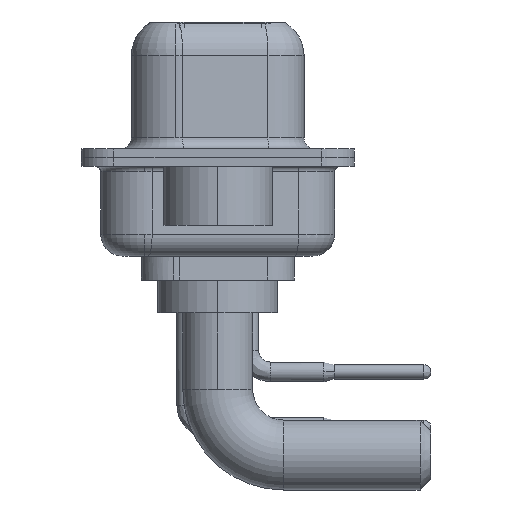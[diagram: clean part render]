
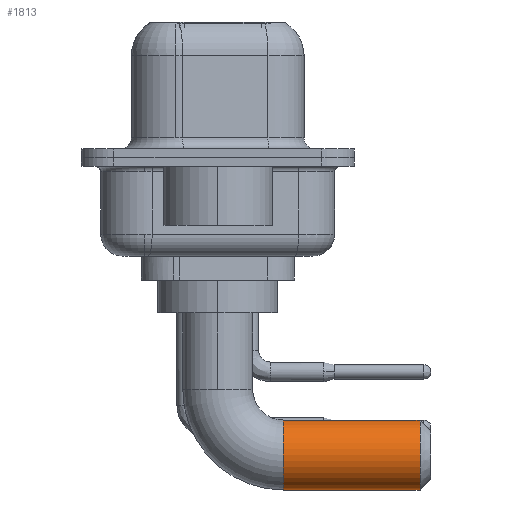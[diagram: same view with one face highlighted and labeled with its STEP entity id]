
A CAD part, left-side view. The second image highlights one B-rep face of the part: STEP entity #1813.
In plain terms, the highlighted cylindrical face has radius 1.6 mm (diameter 3.2 mm), a partial arc.
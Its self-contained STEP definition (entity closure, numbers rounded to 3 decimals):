
#64 = VERTEX_POINT ( 'NONE', #2187 ) ;
#1068 = DIRECTION ( 'NONE',  ( 0., 1., 0. ) ) ;
#1761 = EDGE_CURVE ( 'NONE', #8462, #64, #7492, .T. ) ;
#1813 = ADVANCED_FACE ( 'NONE', ( #10735 ), #24134, .T. ) ;
#2023 = AXIS2_PLACEMENT_3D ( 'NONE', #15691, #21719, #9776 ) ;
#2187 = CARTESIAN_POINT ( 'NONE',  ( 0., -9.25, -4.9 ) ) ;
#3352 = VERTEX_POINT ( 'NONE', #7158 ) ;
#4476 = LINE ( 'NONE', #18139, #21589 ) ;
#4962 = DIRECTION ( 'NONE',  ( 0., 0., -1. ) ) ;
#5904 = ORIENTED_EDGE ( 'NONE', *, *, #1761, .T. ) ;
#6000 = EDGE_CURVE ( 'NONE', #3352, #64, #4476, .T. ) ;
#6040 = VERTEX_POINT ( 'NONE', #10733 ) ;
#6060 = CIRCLE ( 'NONE', #2023, 1.6 ) ;
#7158 = CARTESIAN_POINT ( 'NONE',  ( 0., -3., -4.9 ) ) ;
#7492 = CIRCLE ( 'NONE', #19534, 1.6 ) ;
#8462 = VERTEX_POINT ( 'NONE', #18939 ) ;
#8536 = EDGE_CURVE ( 'NONE', #3352, #6040, #6060, .T. ) ;
#9287 = ORIENTED_EDGE ( 'NONE', *, *, #8536, .T. ) ;
#9776 = DIRECTION ( 'NONE',  ( -1., 0., 0. ) ) ;
#10613 = CARTESIAN_POINT ( 'NONE',  ( 0., -9.25, -6.5 ) ) ;
#10699 = AXIS2_PLACEMENT_3D ( 'NONE', #24014, #23655, #4962 ) ;
#10733 = CARTESIAN_POINT ( 'NONE',  ( 0., -3., -8.1 ) ) ;
#10735 = FACE_OUTER_BOUND ( 'NONE', #18315, .T. ) ;
#10930 = ORIENTED_EDGE ( 'NONE', *, *, #19908, .T. ) ;
#12124 = DIRECTION ( 'NONE',  ( 0., -1., 0. ) ) ;
#15691 = CARTESIAN_POINT ( 'NONE',  ( 0., -3., -6.5 ) ) ;
#17353 = CARTESIAN_POINT ( 'NONE',  ( 0., -3., -8.1 ) ) ;
#17486 = DIRECTION ( 'NONE',  ( 0., -1., 0. ) ) ;
#17920 = VECTOR ( 'NONE', #17486, 1000. ) ;
#18080 = LINE ( 'NONE', #17353, #17920 ) ;
#18139 = CARTESIAN_POINT ( 'NONE',  ( 0., -3., -4.9 ) ) ;
#18315 = EDGE_LOOP ( 'NONE', ( #22514, #9287, #10930, #5904 ) ) ;
#18939 = CARTESIAN_POINT ( 'NONE',  ( 0., -9.25, -8.1 ) ) ;
#19534 = AXIS2_PLACEMENT_3D ( 'NONE', #10613, #1068, #20282 ) ;
#19908 = EDGE_CURVE ( 'NONE', #6040, #8462, #18080, .T. ) ;
#20282 = DIRECTION ( 'NONE',  ( 0., 0., -1. ) ) ;
#21589 = VECTOR ( 'NONE', #12124, 1000. ) ;
#21719 = DIRECTION ( 'NONE',  ( 0., -1., 0. ) ) ;
#22514 = ORIENTED_EDGE ( 'NONE', *, *, #6000, .F. ) ;
#23655 = DIRECTION ( 'NONE',  ( 0., -1., 0. ) ) ;
#24014 = CARTESIAN_POINT ( 'NONE',  ( 0., -3., -6.5 ) ) ;
#24134 = CYLINDRICAL_SURFACE ( 'NONE', #10699, 1.6 ) ;
